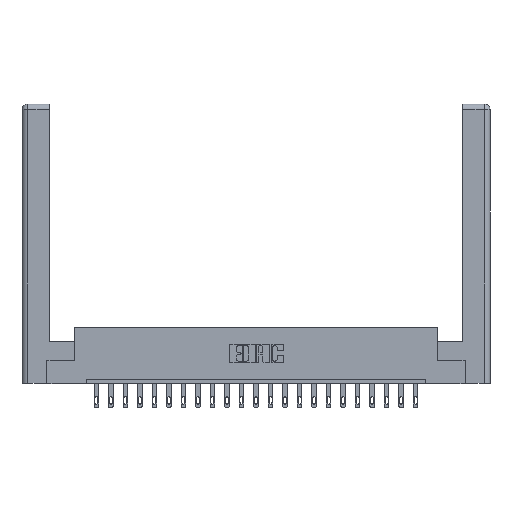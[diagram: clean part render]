
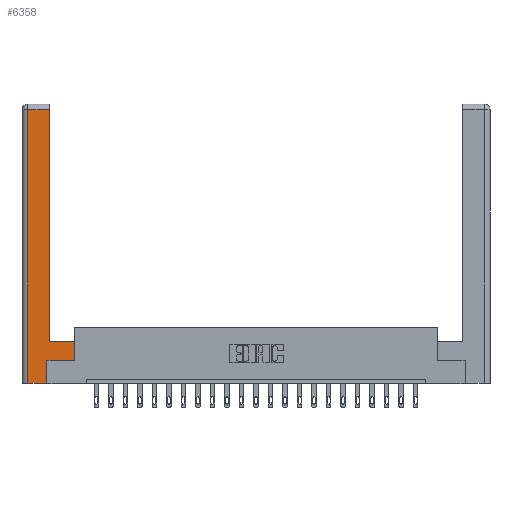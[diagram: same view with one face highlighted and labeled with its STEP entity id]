
A CAD part, top view. The second image highlights one B-rep face of the part: STEP entity #6358.
In plain terms, the highlighted planar face has unit normal (0, 0, 1).
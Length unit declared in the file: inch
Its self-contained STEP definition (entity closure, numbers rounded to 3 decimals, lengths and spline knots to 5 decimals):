
#316 = EDGE_CURVE ( 'NONE', #15109, #16373, #14476, .T. ) ;
#836 = VECTOR ( 'NONE', #15652, 39.37008 ) ;
#994 = EDGE_CURVE ( 'NONE', #8399, #2724, #10668, .T. ) ;
#1377 = CARTESIAN_POINT ( 'NONE',  ( 0.565, 0.245, 0. ) ) ;
#1490 = CARTESIAN_POINT ( 'NONE',  ( 0.265, 0.245, 0. ) ) ;
#1728 = ORIENTED_EDGE ( 'NONE', *, *, #16935, .T. ) ;
#2724 = VERTEX_POINT ( 'NONE', #6192 ) ;
#2866 = EDGE_CURVE ( 'NONE', #7407, #15109, #11386, .T. ) ;
#2887 = CARTESIAN_POINT ( 'NONE',  ( 0.265, 0., 0. ) ) ;
#2922 = CARTESIAN_POINT ( 'NONE',  ( 0.565, 0.45, 0. ) ) ;
#3324 = EDGE_CURVE ( 'NONE', #14753, #8399, #14648, .T. ) ;
#3959 = EDGE_CURVE ( 'NONE', #20216, #14753, #13210, .T. ) ;
#4037 = CARTESIAN_POINT ( 'NONE',  ( 0.565, 0.245, 0. ) ) ;
#4660 = DIRECTION ( 'NONE',  ( 0., 1., 0. ) ) ;
#4692 = DIRECTION ( 'NONE',  ( -1., 0., 0. ) ) ;
#4704 = CARTESIAN_POINT ( 'NONE',  ( 0.295, 0.45, 0. ) ) ;
#4768 = LINE ( 'NONE', #5759, #9548 ) ;
#4927 = ORIENTED_EDGE ( 'NONE', *, *, #994, .T. ) ;
#5179 = VECTOR ( 'NONE', #21888, 39.37008 ) ;
#5759 = CARTESIAN_POINT ( 'NONE',  ( 0.0615, 0., 0. ) ) ;
#6192 = CARTESIAN_POINT ( 'NONE',  ( 0.565, 0.45, 0. ) ) ;
#6204 = ORIENTED_EDGE ( 'NONE', *, *, #3324, .T. ) ;
#6358 = ADVANCED_FACE ( 'NONE', ( #8000 ), #16246, .F. ) ;
#6485 = CARTESIAN_POINT ( 'NONE',  ( 0.295, 3., 0. ) ) ;
#7407 = VERTEX_POINT ( 'NONE', #4704 ) ;
#7642 = EDGE_CURVE ( 'NONE', #16373, #10298, #4768, .T. ) ;
#8000 = FACE_OUTER_BOUND ( 'NONE', #19412, .T. ) ;
#8113 = CARTESIAN_POINT ( 'NONE',  ( 0.0615, 2.94, 0. ) ) ;
#8399 = VERTEX_POINT ( 'NONE', #4037 ) ;
#8478 = CARTESIAN_POINT ( 'NONE',  ( 0.265, 0.245, 0. ) ) ;
#9257 = LINE ( 'NONE', #21737, #18379 ) ;
#9548 = VECTOR ( 'NONE', #21157, 39.37008 ) ;
#10288 = EDGE_CURVE ( 'NONE', #10298, #20216, #17876, .T. ) ;
#10298 = VERTEX_POINT ( 'NONE', #16968 ) ;
#10668 = LINE ( 'NONE', #2922, #21122 ) ;
#10883 = VECTOR ( 'NONE', #16820, 39.37008 ) ;
#11204 = CARTESIAN_POINT ( 'NONE',  ( 0.295, 2.94, 0. ) ) ;
#11386 = LINE ( 'NONE', #6485, #11939 ) ;
#11939 = VECTOR ( 'NONE', #18614, 39.37008 ) ;
#12242 = CARTESIAN_POINT ( 'NONE',  ( 0.0615, 2.94, 0. ) ) ;
#13210 = LINE ( 'NONE', #1490, #5179 ) ;
#14476 = LINE ( 'NONE', #12242, #836 ) ;
#14648 = LINE ( 'NONE', #1377, #22104 ) ;
#14753 = VERTEX_POINT ( 'NONE', #8478 ) ;
#14842 = ORIENTED_EDGE ( 'NONE', *, *, #10288, .T. ) ;
#15109 = VERTEX_POINT ( 'NONE', #11204 ) ;
#15652 = DIRECTION ( 'NONE',  ( -1., 0., 0. ) ) ;
#16246 = PLANE ( 'NONE',  #16886 ) ;
#16373 = VERTEX_POINT ( 'NONE', #8113 ) ;
#16396 = DIRECTION ( 'NONE',  ( -1., 0., 0. ) ) ;
#16820 = DIRECTION ( 'NONE',  ( 1., 0., 0. ) ) ;
#16886 = AXIS2_PLACEMENT_3D ( 'NONE', #21366, #19728, #16396 ) ;
#16935 = EDGE_CURVE ( 'NONE', #2724, #7407, #9257, .T. ) ;
#16968 = CARTESIAN_POINT ( 'NONE',  ( 0.0615, 0., 0. ) ) ;
#17876 = LINE ( 'NONE', #18460, #10883 ) ;
#17957 = ORIENTED_EDGE ( 'NONE', *, *, #2866, .T. ) ;
#17971 = ORIENTED_EDGE ( 'NONE', *, *, #316, .T. ) ;
#18379 = VECTOR ( 'NONE', #4692, 39.37008 ) ;
#18460 = CARTESIAN_POINT ( 'NONE',  ( 0.265, 0., 0. ) ) ;
#18587 = DIRECTION ( 'NONE',  ( 1., 0., 0. ) ) ;
#18614 = DIRECTION ( 'NONE',  ( 0., 1., 0. ) ) ;
#19412 = EDGE_LOOP ( 'NONE', ( #17957, #17971, #21654, #14842, #21656, #6204, #4927, #1728 ) ) ;
#19728 = DIRECTION ( 'NONE',  ( 0., 0., -1. ) ) ;
#20216 = VERTEX_POINT ( 'NONE', #2887 ) ;
#21122 = VECTOR ( 'NONE', #4660, 39.37008 ) ;
#21157 = DIRECTION ( 'NONE',  ( 0., -1., 0. ) ) ;
#21366 = CARTESIAN_POINT ( 'NONE',  ( 0., 0., 0. ) ) ;
#21654 = ORIENTED_EDGE ( 'NONE', *, *, #7642, .T. ) ;
#21656 = ORIENTED_EDGE ( 'NONE', *, *, #3959, .T. ) ;
#21737 = CARTESIAN_POINT ( 'NONE',  ( 0.295, 0.45, 0. ) ) ;
#21888 = DIRECTION ( 'NONE',  ( 0., 1., 0. ) ) ;
#22104 = VECTOR ( 'NONE', #18587, 39.37008 ) ;
